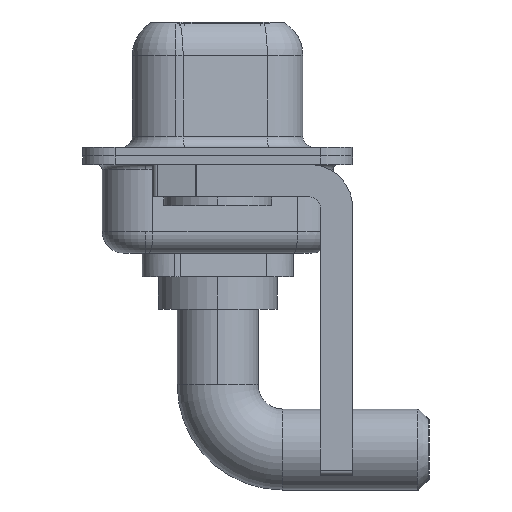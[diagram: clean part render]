
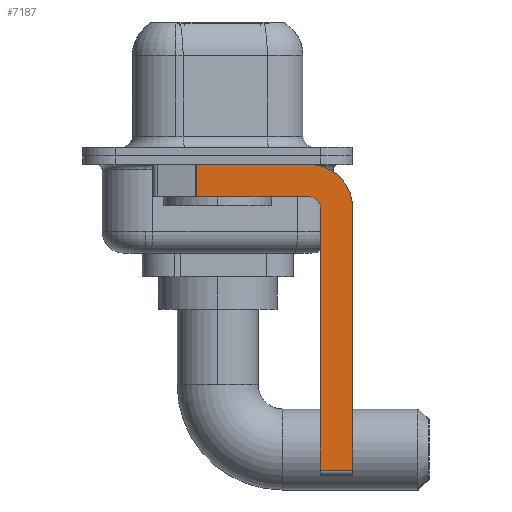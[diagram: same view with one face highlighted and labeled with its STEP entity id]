
A CAD part, left-side view. The second image highlights one B-rep face of the part: STEP entity #7187.
In plain terms, the highlighted planar face has unit normal (-1, 0, 0).
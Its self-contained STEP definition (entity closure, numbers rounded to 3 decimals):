
#30 = EDGE_CURVE ( 'NONE', #947, #727, #7787, .T. ) ;
#727 = VERTEX_POINT ( 'NONE', #3545 ) ;
#733 = CARTESIAN_POINT ( 'NONE',  ( -2.9, -4.75, -14.8 ) ) ;
#897 = CARTESIAN_POINT ( 'NONE',  ( -2.9, -4.25, -1.9 ) ) ;
#947 = VERTEX_POINT ( 'NONE', #897 ) ;
#1017 = ORIENTED_EDGE ( 'NONE', *, *, #6878, .F. ) ;
#1190 = DIRECTION ( 'NONE',  ( -1., 0., 0. ) ) ;
#1213 = CARTESIAN_POINT ( 'NONE',  ( -2.9, 0.978, -0.4 ) ) ;
#1302 = VECTOR ( 'NONE', #6065, 1000. ) ;
#1623 = ORIENTED_EDGE ( 'NONE', *, *, #2886, .F. ) ;
#1839 = CARTESIAN_POINT ( 'NONE',  ( -2.9, -4.25, -2.4 ) ) ;
#2418 = EDGE_CURVE ( 'NONE', #3332, #12067, #10722, .T. ) ;
#2886 = EDGE_CURVE ( 'NONE', #7868, #5542, #5111, .T. ) ;
#2917 = CARTESIAN_POINT ( 'NONE',  ( -2.9, -6.25, -2.4 ) ) ;
#3012 = DIRECTION ( 'NONE',  ( 0., 1., 0. ) ) ;
#3332 = VERTEX_POINT ( 'NONE', #10687 ) ;
#3402 = VECTOR ( 'NONE', #7340, 1000. ) ;
#3427 = AXIS2_PLACEMENT_3D ( 'NONE', #11258, #1190, #7960 ) ;
#3544 = ORIENTED_EDGE ( 'NONE', *, *, #5892, .T. ) ;
#3545 = CARTESIAN_POINT ( 'NONE',  ( -2.9, 0.978, -1.9 ) ) ;
#3661 = EDGE_CURVE ( 'NONE', #12067, #947, #11877, .T. ) ;
#3946 = AXIS2_PLACEMENT_3D ( 'NONE', #1839, #6461, #8456 ) ;
#4118 = FACE_OUTER_BOUND ( 'NONE', #11216, .T. ) ;
#4174 = CARTESIAN_POINT ( 'NONE',  ( -2.9, -6.25, -2.4 ) ) ;
#4806 = DIRECTION ( 'NONE',  ( 0., -1., 0. ) ) ;
#5111 = LINE ( 'NONE', #6142, #1302 ) ;
#5493 = ORIENTED_EDGE ( 'NONE', *, *, #12132, .F. ) ;
#5542 = VERTEX_POINT ( 'NONE', #12801 ) ;
#5567 = LINE ( 'NONE', #10064, #6019 ) ;
#5892 = EDGE_CURVE ( 'NONE', #7868, #727, #5567, .T. ) ;
#6019 = VECTOR ( 'NONE', #9013, 1000. ) ;
#6065 = DIRECTION ( 'NONE',  ( 0., -1., 0. ) ) ;
#6142 = CARTESIAN_POINT ( 'NONE',  ( -2.9, 3., -0.4 ) ) ;
#6184 = VECTOR ( 'NONE', #3012, 1000. ) ;
#6192 = ORIENTED_EDGE ( 'NONE', *, *, #3661, .F. ) ;
#6461 = DIRECTION ( 'NONE',  ( 1., 0., 0. ) ) ;
#6663 = CARTESIAN_POINT ( 'NONE',  ( -2.9, -4.25, -1.9 ) ) ;
#6878 = EDGE_CURVE ( 'NONE', #5542, #7638, #10039, .T. ) ;
#7187 = ADVANCED_FACE ( 'NONE', ( #4118 ), #14200, .F. ) ;
#7340 = DIRECTION ( 'NONE',  ( 0., 0., 1. ) ) ;
#7506 = ORIENTED_EDGE ( 'NONE', *, *, #2418, .F. ) ;
#7638 = VERTEX_POINT ( 'NONE', #4174 ) ;
#7787 = LINE ( 'NONE', #6663, #6184 ) ;
#7868 = VERTEX_POINT ( 'NONE', #1213 ) ;
#7909 = CARTESIAN_POINT ( 'NONE',  ( -2.9, -4.25, -2.4 ) ) ;
#7960 = DIRECTION ( 'NONE',  ( 0., 0., 1. ) ) ;
#8042 = CARTESIAN_POINT ( 'NONE',  ( -2.9, -4.25, -14.55 ) ) ;
#8051 = DIRECTION ( 'NONE',  ( 0., 0., -1. ) ) ;
#8456 = DIRECTION ( 'NONE',  ( 0., 0., -1. ) ) ;
#8647 = CARTESIAN_POINT ( 'NONE',  ( -2.9, -4.75, -2.4 ) ) ;
#8821 = DIRECTION ( 'NONE',  ( 1., 0., 0. ) ) ;
#9013 = DIRECTION ( 'NONE',  ( 0., 0., -1. ) ) ;
#9744 = DIRECTION ( 'NONE',  ( 0., 0., -1. ) ) ;
#9836 = EDGE_CURVE ( 'NONE', #3332, #11274, #11347, .T. ) ;
#9874 = ORIENTED_EDGE ( 'NONE', *, *, #30, .F. ) ;
#10039 = CIRCLE ( 'NONE', #12635, 2. ) ;
#10064 = CARTESIAN_POINT ( 'NONE',  ( -2.9, 0.978, -1.9 ) ) ;
#10365 = VECTOR ( 'NONE', #9744, 1000. ) ;
#10687 = CARTESIAN_POINT ( 'NONE',  ( -2.9, -4.75, -14.55 ) ) ;
#10722 = LINE ( 'NONE', #733, #3402 ) ;
#11052 = VECTOR ( 'NONE', #4806, 1000. ) ;
#11216 = EDGE_LOOP ( 'NONE', ( #1623, #3544, #9874, #6192, #7506, #11383, #5493, #1017 ) ) ;
#11258 = CARTESIAN_POINT ( 'NONE',  ( -2.9, -4.25, -2.4 ) ) ;
#11274 = VERTEX_POINT ( 'NONE', #13108 ) ;
#11347 = LINE ( 'NONE', #8042, #11052 ) ;
#11383 = ORIENTED_EDGE ( 'NONE', *, *, #9836, .T. ) ;
#11877 = CIRCLE ( 'NONE', #3427, 0.5 ) ;
#12067 = VERTEX_POINT ( 'NONE', #8647 ) ;
#12132 = EDGE_CURVE ( 'NONE', #7638, #11274, #13220, .T. ) ;
#12635 = AXIS2_PLACEMENT_3D ( 'NONE', #7909, #8821, #8051 ) ;
#12801 = CARTESIAN_POINT ( 'NONE',  ( -2.9, -4.25, -0.4 ) ) ;
#13108 = CARTESIAN_POINT ( 'NONE',  ( -2.9, -6.25, -14.55 ) ) ;
#13220 = LINE ( 'NONE', #2917, #10365 ) ;
#14200 = PLANE ( 'NONE',  #3946 ) ;
